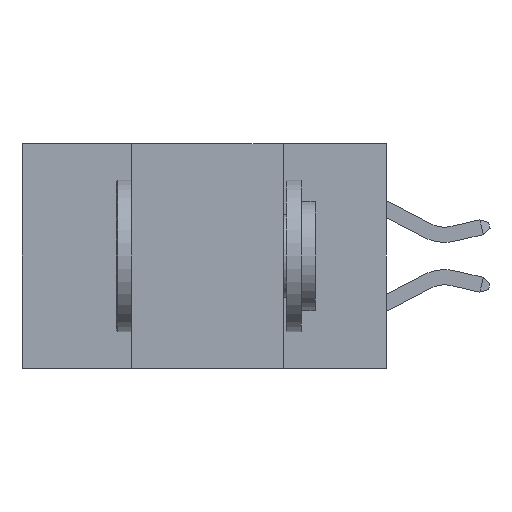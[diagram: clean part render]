
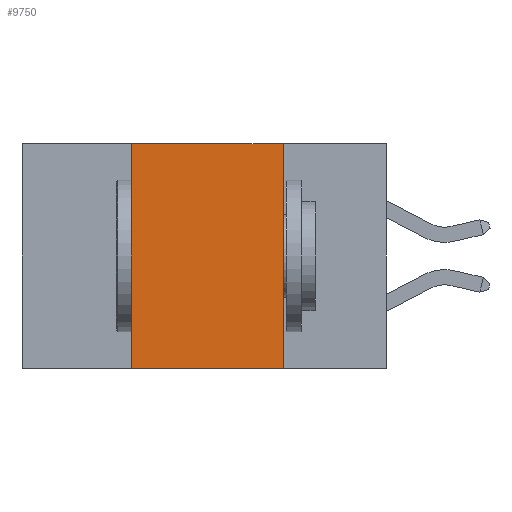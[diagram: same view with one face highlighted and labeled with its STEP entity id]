
A CAD part, left-side view. The second image highlights one B-rep face of the part: STEP entity #9750.
In plain terms, the highlighted planar face has unit normal (-1, 0, 0).
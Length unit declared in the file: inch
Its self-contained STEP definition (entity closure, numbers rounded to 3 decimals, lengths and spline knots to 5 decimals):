
#25 = CARTESIAN_POINT ( 'NONE',  ( 0., 0.17, 0. ) ) ;
#702 = AXIS2_PLACEMENT_3D ( 'NONE', #6322, #3959, #7085 ) ;
#784 = ORIENTED_EDGE ( 'NONE', *, *, #7469, .F. ) ;
#836 = PLANE ( 'NONE',  #702 ) ;
#980 = VERTEX_POINT ( 'NONE', #25 ) ;
#1160 = CARTESIAN_POINT ( 'NONE',  ( 0., 0.17, -0.37 ) ) ;
#1426 = EDGE_LOOP ( 'NONE', ( #784, #6329, #5363, #3511 ) ) ;
#1574 = VECTOR ( 'NONE', #6571, 39.37008 ) ;
#1629 = CARTESIAN_POINT ( 'NONE',  ( 0., 0.42, -0.37 ) ) ;
#2207 = CARTESIAN_POINT ( 'NONE',  ( 0., 0.42, 0. ) ) ;
#2642 = LINE ( 'NONE', #4140, #3940 ) ;
#2661 = EDGE_CURVE ( 'NONE', #9112, #3455, #9481, .T. ) ;
#3455 = VERTEX_POINT ( 'NONE', #2207 ) ;
#3511 = ORIENTED_EDGE ( 'NONE', *, *, #3611, .T. ) ;
#3611 = EDGE_CURVE ( 'NONE', #9112, #7672, #5498, .T. ) ;
#3940 = VECTOR ( 'NONE', #8075, 39.37008 ) ;
#3959 = DIRECTION ( 'NONE',  ( 1., 0., 0. ) ) ;
#4140 = CARTESIAN_POINT ( 'NONE',  ( 0., 0.6, 0. ) ) ;
#4722 = CARTESIAN_POINT ( 'NONE',  ( 0., 0.6, -0.37 ) ) ;
#5363 = ORIENTED_EDGE ( 'NONE', *, *, #2661, .F. ) ;
#5498 = LINE ( 'NONE', #4722, #1574 ) ;
#6254 = DIRECTION ( 'NONE',  ( 0., 0., 1. ) ) ;
#6322 = CARTESIAN_POINT ( 'NONE',  ( 0., 0.6, 0. ) ) ;
#6329 = ORIENTED_EDGE ( 'NONE', *, *, #6439, .F. ) ;
#6439 = EDGE_CURVE ( 'NONE', #3455, #980, #2642, .T. ) ;
#6571 = DIRECTION ( 'NONE',  ( 0., -1., 0. ) ) ;
#7014 = CARTESIAN_POINT ( 'NONE',  ( 0., 0.17, -0.37 ) ) ;
#7085 = DIRECTION ( 'NONE',  ( 0., 0., -1. ) ) ;
#7469 = EDGE_CURVE ( 'NONE', #980, #7672, #9286, .T. ) ;
#7598 = CARTESIAN_POINT ( 'NONE',  ( 0., 0.42, -0.37 ) ) ;
#7672 = VERTEX_POINT ( 'NONE', #1160 ) ;
#7860 = VECTOR ( 'NONE', #6254, 39.37008 ) ;
#8075 = DIRECTION ( 'NONE',  ( 0., -1., 0. ) ) ;
#8390 = DIRECTION ( 'NONE',  ( 0., 0., -1. ) ) ;
#8491 = VECTOR ( 'NONE', #8390, 39.37008 ) ;
#9112 = VERTEX_POINT ( 'NONE', #7598 ) ;
#9286 = LINE ( 'NONE', #7014, #8491 ) ;
#9481 = LINE ( 'NONE', #1629, #7860 ) ;
#9750 = ADVANCED_FACE ( 'NONE', ( #10006 ), #836, .F. ) ;
#10006 = FACE_OUTER_BOUND ( 'NONE', #1426, .T. ) ;
